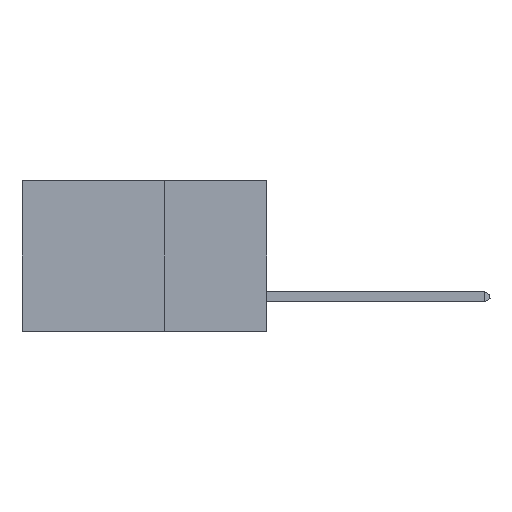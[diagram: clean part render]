
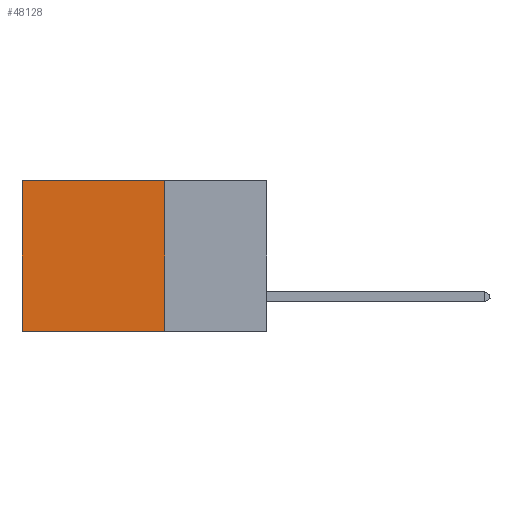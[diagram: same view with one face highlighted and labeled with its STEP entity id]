
A CAD part, left-side view. The second image highlights one B-rep face of the part: STEP entity #48128.
In plain terms, the highlighted planar face has unit normal (-1, 0, 0).
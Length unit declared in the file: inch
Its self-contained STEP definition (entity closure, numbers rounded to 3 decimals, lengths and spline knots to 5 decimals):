
#886 = EDGE_CURVE ( 'NONE', #46317, #1669, #28191, .T. ) ;
#1636 = VECTOR ( 'NONE', #44025, 39.37008 ) ;
#1669 = VERTEX_POINT ( 'NONE', #38482 ) ;
#2428 = FACE_OUTER_BOUND ( 'NONE', #12915, .T. ) ;
#3746 = VECTOR ( 'NONE', #44591, 39.37008 ) ;
#5628 = LINE ( 'NONE', #21562, #41013 ) ;
#7986 = ORIENTED_EDGE ( 'NONE', *, *, #37009, .F. ) ;
#9621 = CARTESIAN_POINT ( 'NONE',  ( 0.2875, 0.6, -0.37 ) ) ;
#11581 = CARTESIAN_POINT ( 'NONE',  ( 0.2875, 0.25, 0. ) ) ;
#12915 = EDGE_LOOP ( 'NONE', ( #31049, #7986, #17914, #27028 ) ) ;
#15521 = DIRECTION ( 'NONE',  ( 0., 0., -1. ) ) ;
#17914 = ORIENTED_EDGE ( 'NONE', *, *, #40857, .F. ) ;
#19150 = VERTEX_POINT ( 'NONE', #9621 ) ;
#19655 = CARTESIAN_POINT ( 'NONE',  ( 0.2875, 0.25, 0. ) ) ;
#20209 = LINE ( 'NONE', #24504, #49562 ) ;
#21562 = CARTESIAN_POINT ( 'NONE',  ( 0.2875, 0.25, 0. ) ) ;
#23823 = EDGE_CURVE ( 'NONE', #1669, #19150, #44171, .T. ) ;
#24504 = CARTESIAN_POINT ( 'NONE',  ( 0.2875, 0.25, -0.37 ) ) ;
#25577 = VERTEX_POINT ( 'NONE', #37389 ) ;
#26214 = DIRECTION ( 'NONE',  ( 0., 0., -1. ) ) ;
#27028 = ORIENTED_EDGE ( 'NONE', *, *, #886, .T. ) ;
#28191 = LINE ( 'NONE', #48079, #3746 ) ;
#31049 = ORIENTED_EDGE ( 'NONE', *, *, #23823, .T. ) ;
#34369 = DIRECTION ( 'NONE',  ( 1., 0., 0. ) ) ;
#34480 = CARTESIAN_POINT ( 'NONE',  ( 0.2875, 0.6, 0. ) ) ;
#37009 = EDGE_CURVE ( 'NONE', #25577, #19150, #20209, .T. ) ;
#37389 = CARTESIAN_POINT ( 'NONE',  ( 0.2875, 0.25, -0.37 ) ) ;
#38141 = AXIS2_PLACEMENT_3D ( 'NONE', #19655, #34369, #15521 ) ;
#38482 = CARTESIAN_POINT ( 'NONE',  ( 0.2875, 0.6, 0. ) ) ;
#40857 = EDGE_CURVE ( 'NONE', #46317, #25577, #5628, .T. ) ;
#41013 = VECTOR ( 'NONE', #26214, 39.37008 ) ;
#43446 = DIRECTION ( 'NONE',  ( 0., 1., 0. ) ) ;
#44025 = DIRECTION ( 'NONE',  ( 0., 0., -1. ) ) ;
#44171 = LINE ( 'NONE', #34480, #1636 ) ;
#44591 = DIRECTION ( 'NONE',  ( 0., 1., 0. ) ) ;
#45812 = PLANE ( 'NONE',  #38141 ) ;
#46317 = VERTEX_POINT ( 'NONE', #11581 ) ;
#48079 = CARTESIAN_POINT ( 'NONE',  ( 0.2875, 0.25, 0. ) ) ;
#48128 = ADVANCED_FACE ( 'NONE', ( #2428 ), #45812, .F. ) ;
#49562 = VECTOR ( 'NONE', #43446, 39.37008 ) ;
